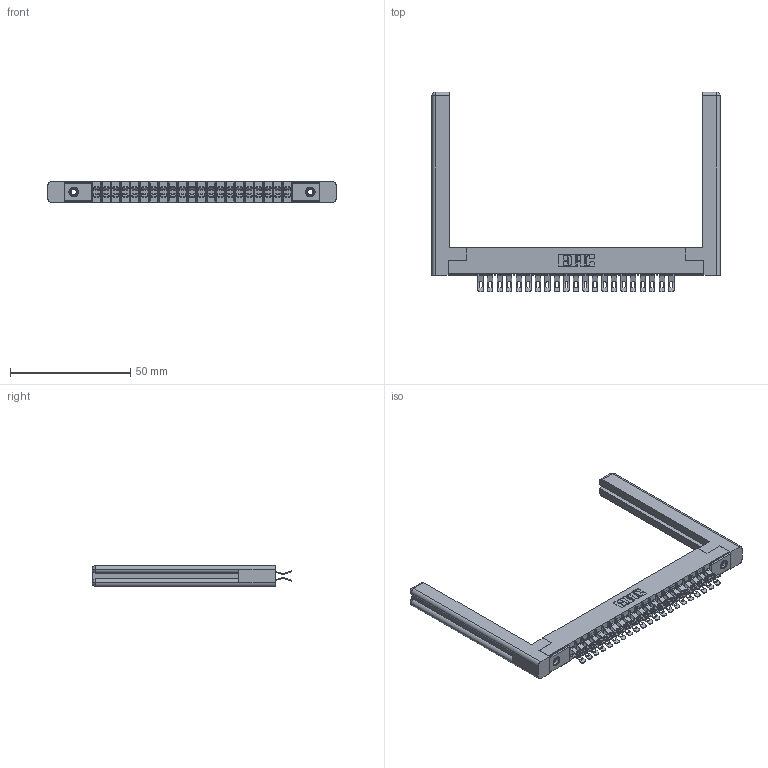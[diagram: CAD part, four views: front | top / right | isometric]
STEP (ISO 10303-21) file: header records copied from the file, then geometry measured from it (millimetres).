
FILE_DESCRIPTION (( 'STEP AP203' ), '1' );
FILE_NAME ('355-042-555-558.STEP', '2019-09-11T13:52:03', ( '' ), ( '' ), 'SwSTEP 2.0', 'SolidWorks 2016', '' );
FILE_SCHEMA (( 'CONFIG_CONTROL_DESIGN' ));
Length unit declared in the file: inch
Products named in the file (5): 307-220-058; 305-290-001_555; 305 Part_.156 Dia; 345-250-001_345-250-001-102; 355-042-555-558
Assembly tree (47 placements, depth 2):
  355-042-555-558
    305 Part_.156 Dia
    305-290-001_555  x42
    345-250-001_345-250-001-102  x2
    307-220-058  x2
Bounding box: 119.84 x 83.06 x 8.71 mm (x, y, z)
Volume: 15070.5 mm3; surface area: 20234.6 mm2
Topology: 47 solids, 47 shells, 3030 faces, 8965 edges, 5850 vertices
Faces by surface type: plane 1496, cylinder 1426, sphere 84, cone 12, torus 12
Entity records: 28551 total; most frequent: CARTESIAN_POINT 4758, ORIENTED_EDGE 4652, DIRECTION 4576, EDGE_CURVE 2326, VECTOR 1828, LINE 1828, VERTEX_POINT 1486, AXIS2_PLACEMENT_3D 1374
